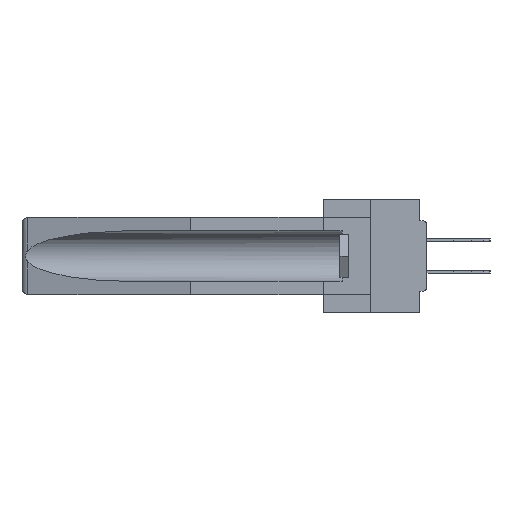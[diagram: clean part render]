
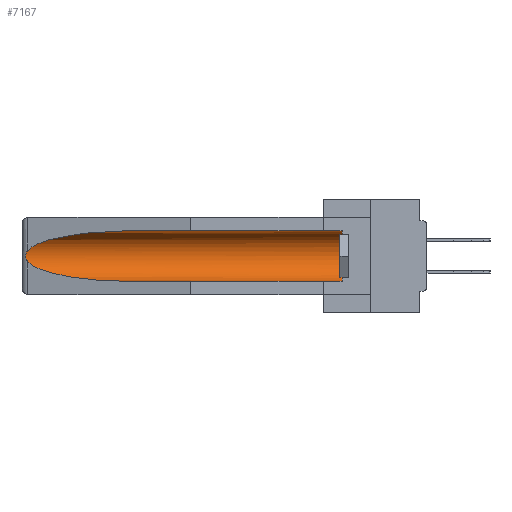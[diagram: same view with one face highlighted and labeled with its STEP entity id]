
A CAD part, left-side view. The second image highlights one B-rep face of the part: STEP entity #7167.
In plain terms, the highlighted cylindrical face has radius 2.857 mm (diameter 5.715 mm), a partial arc.
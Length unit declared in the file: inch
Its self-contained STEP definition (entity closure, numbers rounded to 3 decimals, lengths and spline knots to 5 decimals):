
#256 = LINE ( 'NONE', #4485, #11837 ) ;
#465 = CARTESIAN_POINT ( 'NONE',  ( 0.26537, 1.52718, -0.19328 ) ) ;
#1386 = DIRECTION ( 'NONE',  ( 0., 0., 1. ) ) ;
#2086 = ORIENTED_EDGE ( 'NONE', *, *, #4207, .T. ) ;
#2468 = CARTESIAN_POINT ( 'NONE',  ( 0.26537, 1.52718, -0.14972 ) ) ;
#2671 = VERTEX_POINT ( 'NONE', #31723 ) ;
#3160 = DIRECTION ( 'NONE',  ( 0., 1., 0. ) ) ;
#3433 = CARTESIAN_POINT ( 'NONE',  ( 0.155, 1.07973, -0.284 ) ) ;
#4207 = EDGE_CURVE ( 'NONE', #31102, #35102, #10201, .T. ) ;
#4485 = CARTESIAN_POINT ( 'NONE',  ( 0.155, -0.30754, -0.284 ) ) ;
#5080 = FACE_OUTER_BOUND ( 'NONE', #31070, .T. ) ;
#5659 = CARTESIAN_POINT ( 'NONE',  ( 0.2673, 1.53269, -0.17917 ) ) ;
#6611 = AXIS2_PLACEMENT_3D ( 'NONE', #36718, #15893, #1386 ) ;
#7167 = ADVANCED_FACE ( 'NONE', ( #5080 ), #14771, .F. ) ;
#8623 = CARTESIAN_POINT ( 'NONE',  ( 0.26537, 1.52718, -0.14972 ) ) ;
#9310 = VERTEX_POINT ( 'NONE', #12583 ) ;
#9396 = CARTESIAN_POINT ( 'NONE',  ( 0.26537, 1.52718, -0.19328 ) ) ;
#10201 = B_SPLINE_CURVE_WITH_KNOTS ( 'NONE', 3,
 ( #8623, #35010, #26228, #20402, #37989, #20260, #5659, #29343, #11598, #11467 ),
 .UNSPECIFIED., .F., .F.,
 ( 4, 2, 2, 2, 4 ),
 ( 0., 0.00029, 0.00058, 0.00087, 0.00117 ),
 .UNSPECIFIED. ) ;
#11467 = CARTESIAN_POINT ( 'NONE',  ( 0.26537, 1.52718, -0.19328 ) ) ;
#11598 = CARTESIAN_POINT ( 'NONE',  ( 0.26597, 1.5296, -0.19026 ) ) ;
#11837 = VECTOR ( 'NONE', #33632, 39.37008 ) ;
#11876 =( BOUNDED_CURVE ( )  B_SPLINE_CURVE ( 3, ( #465, #32974, #26998, #3433 ),
 .UNSPECIFIED., .F., .F. ) 
 B_SPLINE_CURVE_WITH_KNOTS ( ( 4, 4 ),
 ( 0.1948, 1.5708 ),
 .UNSPECIFIED. ) 
 CURVE ( )  GEOMETRIC_REPRESENTATION_ITEM ( )  RATIONAL_B_SPLINE_CURVE ( ( 1., 0.848, 0.848, 1. ) ) 
 REPRESENTATION_ITEM ( '' )  );
#12583 = CARTESIAN_POINT ( 'NONE',  ( 0.155, 1.07973, -0.059 ) ) ;
#13054 = CIRCLE ( 'NONE', #6611, 0.1125 ) ;
#14644 = ORIENTED_EDGE ( 'NONE', *, *, #22068, .T. ) ;
#14771 = CYLINDRICAL_SURFACE ( 'NONE', #37034, 0.1125 ) ;
#15893 = DIRECTION ( 'NONE',  ( 0., -1., 0. ) ) ;
#16708 = ORIENTED_EDGE ( 'NONE', *, *, #30178, .F. ) ;
#17703 = DIRECTION ( 'NONE',  ( 0., 0., 1. ) ) ;
#18333 = EDGE_CURVE ( 'NONE', #24639, #30910, #13054, .T. ) ;
#18339 = CARTESIAN_POINT ( 'NONE',  ( 0.26537, 1.52718, -0.14972 ) ) ;
#18471 = CARTESIAN_POINT ( 'NONE',  ( 0.21114, 1.30732, -0.059 ) ) ;
#20114 = LINE ( 'NONE', #33070, #25221 ) ;
#20260 = CARTESIAN_POINT ( 'NONE',  ( 0.2675, 1.53308, -0.17534 ) ) ;
#20402 = CARTESIAN_POINT ( 'NONE',  ( 0.2673, 1.5327, -0.16383 ) ) ;
#22068 = EDGE_CURVE ( 'NONE', #30910, #9310, #20114, .T. ) ;
#23431 = ORIENTED_EDGE ( 'NONE', *, *, #35024, .T. ) ;
#24639 = VERTEX_POINT ( 'NONE', #35449 ) ;
#24987 = ORIENTED_EDGE ( 'NONE', *, *, #18333, .T. ) ;
#25221 = VECTOR ( 'NONE', #26981, 39.37008 ) ;
#26190 = ORIENTED_EDGE ( 'NONE', *, *, #32399, .T. ) ;
#26228 = CARTESIAN_POINT ( 'NONE',  ( 0.26654, 1.53092, -0.15636 ) ) ;
#26981 = DIRECTION ( 'NONE',  ( 0., 1., 0. ) ) ;
#26998 = CARTESIAN_POINT ( 'NONE',  ( 0.21114, 1.30732, -0.284 ) ) ;
#29329 = CARTESIAN_POINT ( 'NONE',  ( 0.155, -0.30754, -0.1715 ) ) ;
#29343 = CARTESIAN_POINT ( 'NONE',  ( 0.26655, 1.53094, -0.18657 ) ) ;
#29983 = CARTESIAN_POINT ( 'NONE',  ( 0.25451, 1.48313, -0.09465 ) ) ;
#30178 = EDGE_CURVE ( 'NONE', #24639, #2671, #256, .T. ) ;
#30910 = VERTEX_POINT ( 'NONE', #31884 ) ;
#31070 = EDGE_LOOP ( 'NONE', ( #23431, #2086, #26190, #16708, #24987, #14644 ) ) ;
#31102 = VERTEX_POINT ( 'NONE', #2468 ) ;
#31723 = CARTESIAN_POINT ( 'NONE',  ( 0.155, 1.07973, -0.284 ) ) ;
#31884 = CARTESIAN_POINT ( 'NONE',  ( 0.155, 0.126, -0.059 ) ) ;
#32399 = EDGE_CURVE ( 'NONE', #35102, #2671, #11876, .T. ) ;
#32974 = CARTESIAN_POINT ( 'NONE',  ( 0.25451, 1.48313, -0.24835 ) ) ;
#33070 = CARTESIAN_POINT ( 'NONE',  ( 0.155, -0.30754, -0.059 ) ) ;
#33632 = DIRECTION ( 'NONE',  ( 0., 1., 0. ) ) ;
#35010 = CARTESIAN_POINT ( 'NONE',  ( 0.26597, 1.52961, -0.15275 ) ) ;
#35024 = EDGE_CURVE ( 'NONE', #9310, #31102, #35844, .T. ) ;
#35102 = VERTEX_POINT ( 'NONE', #9396 ) ;
#35449 = CARTESIAN_POINT ( 'NONE',  ( 0.155, 0.126, -0.284 ) ) ;
#35844 =( BOUNDED_CURVE ( )  B_SPLINE_CURVE ( 3, ( #36039, #18471, #29983, #18339 ),
 .UNSPECIFIED., .F., .F. ) 
 B_SPLINE_CURVE_WITH_KNOTS ( ( 4, 4 ),
 ( 4.71239, 6.08839 ),
 .UNSPECIFIED. ) 
 CURVE ( )  GEOMETRIC_REPRESENTATION_ITEM ( )  RATIONAL_B_SPLINE_CURVE ( ( 1., 0.848, 0.848, 1. ) ) 
 REPRESENTATION_ITEM ( '' )  );
#36039 = CARTESIAN_POINT ( 'NONE',  ( 0.155, 1.07973, -0.059 ) ) ;
#36718 = CARTESIAN_POINT ( 'NONE',  ( 0.155, 0.126, -0.1715 ) ) ;
#37034 = AXIS2_PLACEMENT_3D ( 'NONE', #29329, #3160, #17703 ) ;
#37989 = CARTESIAN_POINT ( 'NONE',  ( 0.2675, 1.53308, -0.16763 ) ) ;
